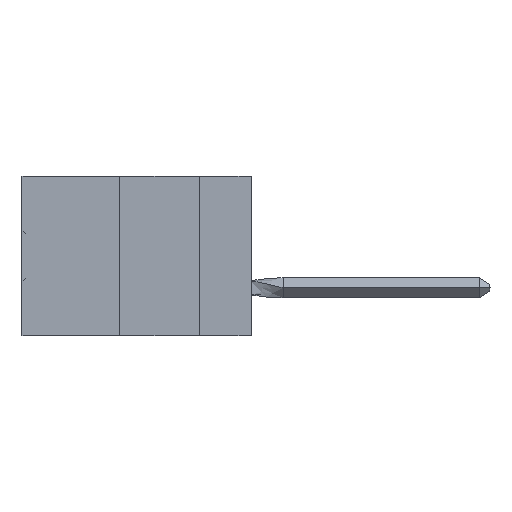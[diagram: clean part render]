
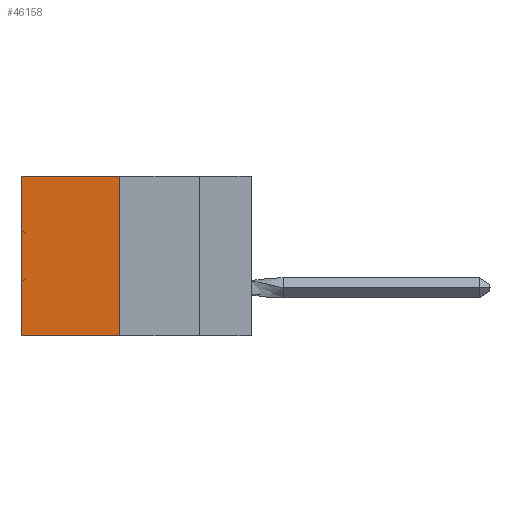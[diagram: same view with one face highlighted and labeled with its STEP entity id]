
A CAD part, left-side view. The second image highlights one B-rep face of the part: STEP entity #46158.
In plain terms, the highlighted planar face has unit normal (-1, 0, 0).
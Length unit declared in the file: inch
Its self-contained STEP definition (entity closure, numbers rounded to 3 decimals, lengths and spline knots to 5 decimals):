
#716 = CARTESIAN_POINT ( 'NONE',  ( 0.305, 0.72, -0.5 ) ) ;
#2561 = ORIENTED_EDGE ( 'NONE', *, *, #18507, .T. ) ;
#2761 = DIRECTION ( 'NONE',  ( 0., 0., -1. ) ) ;
#7002 = EDGE_CURVE ( 'NONE', #34638, #47650, #26000, .T. ) ;
#8589 = LINE ( 'NONE', #28370, #36404 ) ;
#13031 = ORIENTED_EDGE ( 'NONE', *, *, #29119, .F. ) ;
#13480 = VECTOR ( 'NONE', #2761, 39.37008 ) ;
#16077 = FACE_OUTER_BOUND ( 'NONE', #39407, .T. ) ;
#16453 = AXIS2_PLACEMENT_3D ( 'NONE', #56442, #23546, #41794 ) ;
#18507 = EDGE_CURVE ( 'NONE', #34638, #39669, #19330, .T. ) ;
#18777 = ORIENTED_EDGE ( 'NONE', *, *, #7002, .F. ) ;
#19330 = LINE ( 'NONE', #19865, #59768 ) ;
#19854 = CARTESIAN_POINT ( 'NONE',  ( 0.305, 0.413, 0. ) ) ;
#19865 = CARTESIAN_POINT ( 'NONE',  ( 0.305, 0.413, 0. ) ) ;
#23546 = DIRECTION ( 'NONE',  ( 1., 0., 0. ) ) ;
#25535 = VECTOR ( 'NONE', #28905, 39.37008 ) ;
#26000 = LINE ( 'NONE', #26500, #13480 ) ;
#26500 = CARTESIAN_POINT ( 'NONE',  ( 0.305, 0.413, -0.5 ) ) ;
#28370 = CARTESIAN_POINT ( 'NONE',  ( 0.305, 0.72, -0.5 ) ) ;
#28905 = DIRECTION ( 'NONE',  ( 0., 1., 0. ) ) ;
#29119 = EDGE_CURVE ( 'NONE', #47650, #39551, #50511, .T. ) ;
#29689 = EDGE_CURVE ( 'NONE', #39669, #39551, #8589, .T. ) ;
#34638 = VERTEX_POINT ( 'NONE', #19854 ) ;
#36404 = VECTOR ( 'NONE', #51824, 39.37008 ) ;
#39407 = EDGE_LOOP ( 'NONE', ( #53479, #13031, #18777, #2561 ) ) ;
#39551 = VERTEX_POINT ( 'NONE', #716 ) ;
#39669 = VERTEX_POINT ( 'NONE', #55627 ) ;
#41607 = CARTESIAN_POINT ( 'NONE',  ( 0.305, 0.413, -0.5 ) ) ;
#41794 = DIRECTION ( 'NONE',  ( 0., 0., -1. ) ) ;
#46158 = ADVANCED_FACE ( 'NONE', ( #16077 ), #52147, .F. ) ;
#47613 = DIRECTION ( 'NONE',  ( 0., 1., 0. ) ) ;
#47650 = VERTEX_POINT ( 'NONE', #54598 ) ;
#50511 = LINE ( 'NONE', #41607, #25535 ) ;
#51824 = DIRECTION ( 'NONE',  ( 0., 0., -1. ) ) ;
#52147 = PLANE ( 'NONE',  #16453 ) ;
#53479 = ORIENTED_EDGE ( 'NONE', *, *, #29689, .T. ) ;
#54598 = CARTESIAN_POINT ( 'NONE',  ( 0.305, 0.413, -0.5 ) ) ;
#55627 = CARTESIAN_POINT ( 'NONE',  ( 0.305, 0.72, 0. ) ) ;
#56442 = CARTESIAN_POINT ( 'NONE',  ( 0.305, 0.413, -0.5 ) ) ;
#59768 = VECTOR ( 'NONE', #47613, 39.37008 ) ;
